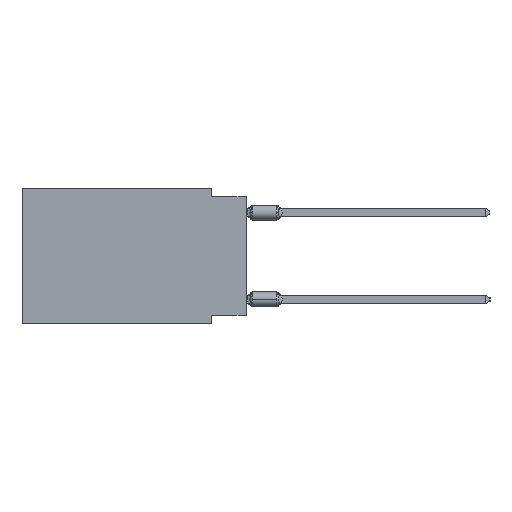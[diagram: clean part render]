
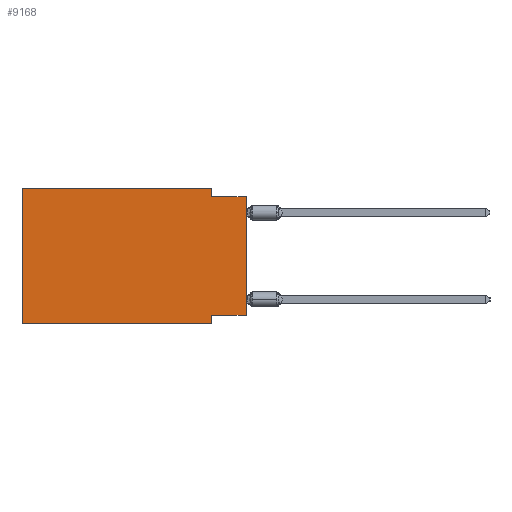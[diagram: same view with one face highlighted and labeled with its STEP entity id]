
A CAD part, left-side view. The second image highlights one B-rep face of the part: STEP entity #9168.
In plain terms, the highlighted planar face has unit normal (-1, 0, 0).
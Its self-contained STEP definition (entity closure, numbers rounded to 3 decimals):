
#394 = VECTOR ( 'NONE', #45826, 1000. ) ;
#573 = EDGE_CURVE ( 'NONE', #21630, #32880, #18413, .T. ) ;
#1763 = CARTESIAN_POINT ( 'NONE',  ( 0., 2.54, -9.906 ) ) ;
#4993 = ORIENTED_EDGE ( 'NONE', *, *, #573, .T. ) ;
#5440 = LINE ( 'NONE', #14785, #27435 ) ;
#6784 = CARTESIAN_POINT ( 'NONE',  ( 0., 16.383, -9.906 ) ) ;
#9077 = CARTESIAN_POINT ( 'NONE',  ( 0., 16.383, 0. ) ) ;
#9168 = ADVANCED_FACE ( 'NONE', ( #33735 ), #11502, .F. ) ;
#9335 = LINE ( 'NONE', #50247, #14684 ) ;
#9515 = VERTEX_POINT ( 'NONE', #26513 ) ;
#9636 = CARTESIAN_POINT ( 'NONE',  ( 0., 16.383, -9.906 ) ) ;
#10811 = DIRECTION ( 'NONE',  ( 0., 0., -1. ) ) ;
#11483 = VERTEX_POINT ( 'NONE', #26090 ) ;
#11502 = PLANE ( 'NONE',  #55089 ) ;
#14495 = DIRECTION ( 'NONE',  ( 0., -1., 0. ) ) ;
#14565 = EDGE_CURVE ( 'NONE', #21630, #11483, #44450, .T. ) ;
#14684 = VECTOR ( 'NONE', #23943, 1000. ) ;
#14785 = CARTESIAN_POINT ( 'NONE',  ( 0., 16.383, 0. ) ) ;
#15595 = DIRECTION ( 'NONE',  ( 1., 0., 0. ) ) ;
#15982 = DIRECTION ( 'NONE',  ( 0., -1., 0. ) ) ;
#16971 = ORIENTED_EDGE ( 'NONE', *, *, #14565, .F. ) ;
#17639 = CARTESIAN_POINT ( 'NONE',  ( 0., 2.54, -9.271 ) ) ;
#17833 = DIRECTION ( 'NONE',  ( 0., -1., 0. ) ) ;
#18099 = EDGE_CURVE ( 'NONE', #35668, #32880, #28392, .T. ) ;
#18284 = VERTEX_POINT ( 'NONE', #45849 ) ;
#18342 = CARTESIAN_POINT ( 'NONE',  ( 0., 0., 0. ) ) ;
#18413 = LINE ( 'NONE', #9636, #49770 ) ;
#18679 = ORIENTED_EDGE ( 'NONE', *, *, #20847, .F. ) ;
#19159 = ORIENTED_EDGE ( 'NONE', *, *, #49103, .T. ) ;
#19399 = VECTOR ( 'NONE', #47810, 1000. ) ;
#20293 = DIRECTION ( 'NONE',  ( 0., 0., -1. ) ) ;
#20587 = ORIENTED_EDGE ( 'NONE', *, *, #29115, .F. ) ;
#20847 = EDGE_CURVE ( 'NONE', #18284, #9515, #9335, .T. ) ;
#21630 = VERTEX_POINT ( 'NONE', #6784 ) ;
#22837 = DIRECTION ( 'NONE',  ( 0., 0., 1. ) ) ;
#23943 = DIRECTION ( 'NONE',  ( 0., 0., -1. ) ) ;
#24476 = CARTESIAN_POINT ( 'NONE',  ( 0., 0., -0.635 ) ) ;
#26090 = CARTESIAN_POINT ( 'NONE',  ( 0., 16.383, 0. ) ) ;
#26513 = CARTESIAN_POINT ( 'NONE',  ( 0., 2.54, -0.635 ) ) ;
#27195 = CARTESIAN_POINT ( 'NONE',  ( 0., 2.54, -9.906 ) ) ;
#27435 = VECTOR ( 'NONE', #14495, 1000. ) ;
#28002 = LINE ( 'NONE', #18342, #394 ) ;
#28392 = LINE ( 'NONE', #1763, #37059 ) ;
#29115 = EDGE_CURVE ( 'NONE', #11483, #18284, #5440, .T. ) ;
#31857 = CARTESIAN_POINT ( 'NONE',  ( 0., 0., -9.271 ) ) ;
#32880 = VERTEX_POINT ( 'NONE', #27195 ) ;
#33127 = CARTESIAN_POINT ( 'NONE',  ( 0., 0., -0.635 ) ) ;
#33735 = FACE_OUTER_BOUND ( 'NONE', #35033, .T. ) ;
#33981 = EDGE_CURVE ( 'NONE', #45355, #35668, #53069, .T. ) ;
#35033 = EDGE_LOOP ( 'NONE', ( #19159, #35136, #18679, #20587, #16971, #4993, #49469, #47198 ) ) ;
#35136 = ORIENTED_EDGE ( 'NONE', *, *, #49302, .F. ) ;
#35668 = VERTEX_POINT ( 'NONE', #17639 ) ;
#37059 = VECTOR ( 'NONE', #10811, 1000. ) ;
#40514 = VERTEX_POINT ( 'NONE', #33127 ) ;
#43182 = VECTOR ( 'NONE', #22837, 1000. ) ;
#44450 = LINE ( 'NONE', #9077, #43182 ) ;
#45355 = VERTEX_POINT ( 'NONE', #31857 ) ;
#45826 = DIRECTION ( 'NONE',  ( 0., 0., 1. ) ) ;
#45849 = CARTESIAN_POINT ( 'NONE',  ( 0., 2.54, 0. ) ) ;
#47198 = ORIENTED_EDGE ( 'NONE', *, *, #33981, .F. ) ;
#47244 = LINE ( 'NONE', #24476, #56408 ) ;
#47810 = DIRECTION ( 'NONE',  ( 0., 1., 0. ) ) ;
#48679 = CARTESIAN_POINT ( 'NONE',  ( 0., 0., -9.271 ) ) ;
#49103 = EDGE_CURVE ( 'NONE', #45355, #40514, #28002, .T. ) ;
#49302 = EDGE_CURVE ( 'NONE', #9515, #40514, #47244, .T. ) ;
#49469 = ORIENTED_EDGE ( 'NONE', *, *, #18099, .F. ) ;
#49770 = VECTOR ( 'NONE', #17833, 1000. ) ;
#50247 = CARTESIAN_POINT ( 'NONE',  ( 0., 2.54, 0. ) ) ;
#53069 = LINE ( 'NONE', #48679, #19399 ) ;
#55089 = AXIS2_PLACEMENT_3D ( 'NONE', #56230, #15595, #20293 ) ;
#56230 = CARTESIAN_POINT ( 'NONE',  ( 0., 16.383, 0. ) ) ;
#56408 = VECTOR ( 'NONE', #15982, 1000. ) ;
